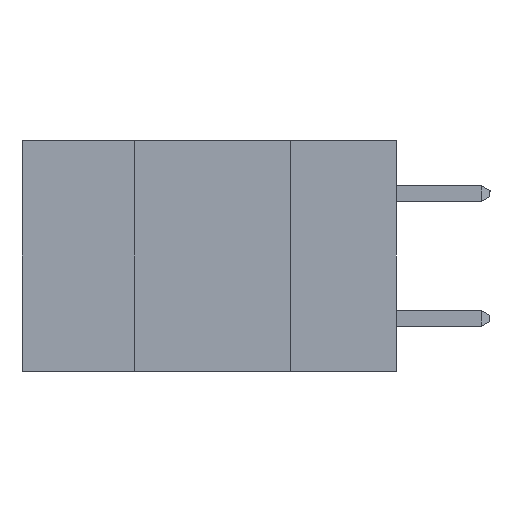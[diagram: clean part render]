
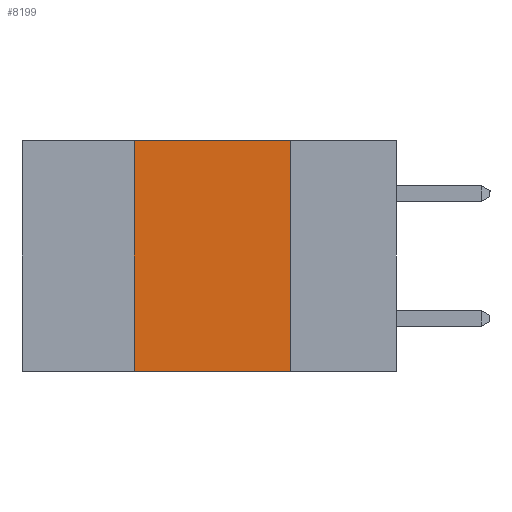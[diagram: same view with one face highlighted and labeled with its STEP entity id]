
A CAD part, left-side view. The second image highlights one B-rep face of the part: STEP entity #8199.
In plain terms, the highlighted planar face has unit normal (-1, 0, 0).
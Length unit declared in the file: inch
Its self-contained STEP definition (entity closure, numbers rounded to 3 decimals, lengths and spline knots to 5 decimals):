
#636 = CARTESIAN_POINT ( 'NONE',  ( 0., 0.42, 0. ) ) ;
#725 = DIRECTION ( 'NONE',  ( 0., -1., 0. ) ) ;
#1215 = VECTOR ( 'NONE', #725, 39.37008 ) ;
#1364 = LINE ( 'NONE', #13519, #25398 ) ;
#1576 = DIRECTION ( 'NONE',  ( 0., 0., -1. ) ) ;
#2679 = DIRECTION ( 'NONE',  ( 0., 0., 1. ) ) ;
#2719 = CARTESIAN_POINT ( 'NONE',  ( 0., 0.6, -0.37 ) ) ;
#2969 = AXIS2_PLACEMENT_3D ( 'NONE', #22562, #20549, #10481 ) ;
#3475 = ORIENTED_EDGE ( 'NONE', *, *, #18924, .F. ) ;
#3614 = DIRECTION ( 'NONE',  ( 0., -1., 0. ) ) ;
#6395 = PLANE ( 'NONE',  #2969 ) ;
#6953 = VERTEX_POINT ( 'NONE', #12811 ) ;
#8099 = CARTESIAN_POINT ( 'NONE',  ( 0., 0.17, -0.37 ) ) ;
#8199 = ADVANCED_FACE ( 'NONE', ( #16440 ), #6395, .F. ) ;
#9013 = EDGE_CURVE ( 'NONE', #17721, #22356, #17123, .T. ) ;
#9639 = LINE ( 'NONE', #25569, #16384 ) ;
#10481 = DIRECTION ( 'NONE',  ( 0., 0., -1. ) ) ;
#11488 = LINE ( 'NONE', #24818, #19030 ) ;
#12811 = CARTESIAN_POINT ( 'NONE',  ( 0., 0.17, 0. ) ) ;
#13519 = CARTESIAN_POINT ( 'NONE',  ( 0., 0.6, 0. ) ) ;
#15390 = ORIENTED_EDGE ( 'NONE', *, *, #22196, .F. ) ;
#16384 = VECTOR ( 'NONE', #1576, 39.37008 ) ;
#16440 = FACE_OUTER_BOUND ( 'NONE', #22076, .T. ) ;
#17123 = LINE ( 'NONE', #2719, #1215 ) ;
#17721 = VERTEX_POINT ( 'NONE', #21633 ) ;
#18861 = ORIENTED_EDGE ( 'NONE', *, *, #22490, .F. ) ;
#18924 = EDGE_CURVE ( 'NONE', #6953, #22356, #9639, .T. ) ;
#19030 = VECTOR ( 'NONE', #2679, 39.37008 ) ;
#19177 = VERTEX_POINT ( 'NONE', #636 ) ;
#20549 = DIRECTION ( 'NONE',  ( 1., 0., 0. ) ) ;
#21462 = ORIENTED_EDGE ( 'NONE', *, *, #9013, .T. ) ;
#21633 = CARTESIAN_POINT ( 'NONE',  ( 0., 0.42, -0.37 ) ) ;
#22076 = EDGE_LOOP ( 'NONE', ( #3475, #15390, #18861, #21462 ) ) ;
#22196 = EDGE_CURVE ( 'NONE', #19177, #6953, #1364, .T. ) ;
#22356 = VERTEX_POINT ( 'NONE', #8099 ) ;
#22490 = EDGE_CURVE ( 'NONE', #17721, #19177, #11488, .T. ) ;
#22562 = CARTESIAN_POINT ( 'NONE',  ( 0., 0.6, 0. ) ) ;
#24818 = CARTESIAN_POINT ( 'NONE',  ( 0., 0.42, -0.37 ) ) ;
#25398 = VECTOR ( 'NONE', #3614, 39.37008 ) ;
#25569 = CARTESIAN_POINT ( 'NONE',  ( 0., 0.17, -0.37 ) ) ;
